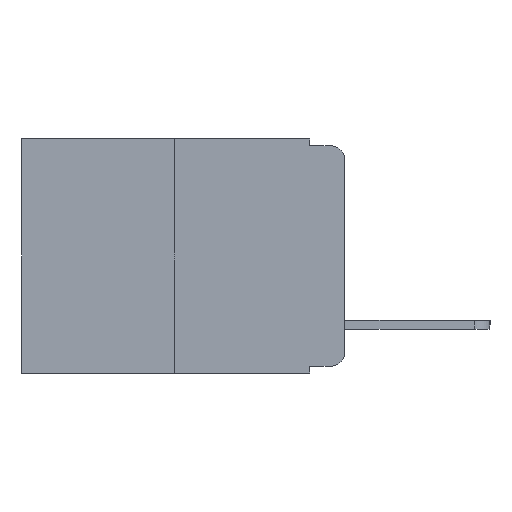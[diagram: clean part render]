
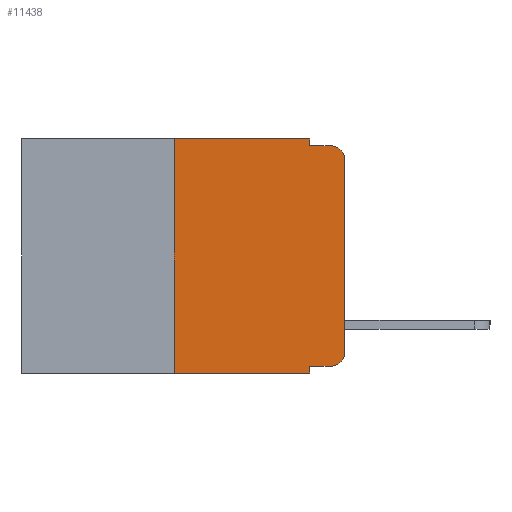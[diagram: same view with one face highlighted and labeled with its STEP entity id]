
A CAD part, left-side view. The second image highlights one B-rep face of the part: STEP entity #11438.
In plain terms, the highlighted planar face has unit normal (-1, 0, 0).
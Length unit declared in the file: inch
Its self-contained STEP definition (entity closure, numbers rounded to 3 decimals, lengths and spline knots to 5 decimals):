
#433 = VECTOR ( 'NONE', #11348, 39.37008 ) ;
#509 = EDGE_CURVE ( 'NONE', #7870, #17186, #17037, .T. ) ;
#562 = DIRECTION ( 'NONE',  ( 1., 0., 0. ) ) ;
#704 = CIRCLE ( 'NONE', #13982, 0.02 ) ;
#1509 = ORIENTED_EDGE ( 'NONE', *, *, #8941, .T. ) ;
#1517 = CARTESIAN_POINT ( 'NONE',  ( 0., 0.02, -0.01 ) ) ;
#1618 = VERTEX_POINT ( 'NONE', #3531 ) ;
#2184 = EDGE_CURVE ( 'NONE', #19096, #15595, #4256, .T. ) ;
#2338 = LINE ( 'NONE', #8220, #433 ) ;
#2557 = CIRCLE ( 'NONE', #18669, 0.02 ) ;
#2660 = ORIENTED_EDGE ( 'NONE', *, *, #10754, .T. ) ;
#2706 = DIRECTION ( 'NONE',  ( 0., 0., -1. ) ) ;
#2711 = DIRECTION ( 'NONE',  ( 0., -1., 0. ) ) ;
#2791 = DIRECTION ( 'NONE',  ( 0., 0., 1. ) ) ;
#3133 = CARTESIAN_POINT ( 'NONE',  ( 0., 0.02, -0.333 ) ) ;
#3222 = ORIENTED_EDGE ( 'NONE', *, *, #9982, .F. ) ;
#3231 = EDGE_LOOP ( 'NONE', ( #7113, #1509, #3222, #7256, #16178, #8993, #17573, #10993, #18399, #2660 ) ) ;
#3531 = CARTESIAN_POINT ( 'NONE',  ( 0., 0.25, 0. ) ) ;
#3757 = DIRECTION ( 'NONE',  ( -1., 0., 0. ) ) ;
#3844 = CARTESIAN_POINT ( 'NONE',  ( 0., 0., -0.313 ) ) ;
#4164 = CARTESIAN_POINT ( 'NONE',  ( 0., 0.051, 0. ) ) ;
#4256 = LINE ( 'NONE', #4164, #17689 ) ;
#5127 = CARTESIAN_POINT ( 'NONE',  ( 0., 0.051, -0.333 ) ) ;
#5367 = VECTOR ( 'NONE', #2711, 39.37008 ) ;
#5397 = DIRECTION ( 'NONE',  ( 0., 0., -1. ) ) ;
#5529 = VERTEX_POINT ( 'NONE', #8472 ) ;
#5745 = DIRECTION ( 'NONE',  ( 0., -1., 0. ) ) ;
#5882 = CARTESIAN_POINT ( 'NONE',  ( 0., 0.473, -0.343 ) ) ;
#6227 = EDGE_CURVE ( 'NONE', #19096, #7724, #18229, .T. ) ;
#6807 = PLANE ( 'NONE',  #12780 ) ;
#7066 = LINE ( 'NONE', #5882, #7161 ) ;
#7113 = ORIENTED_EDGE ( 'NONE', *, *, #8468, .T. ) ;
#7161 = VECTOR ( 'NONE', #17701, 39.37008 ) ;
#7256 = ORIENTED_EDGE ( 'NONE', *, *, #509, .F. ) ;
#7286 = EDGE_CURVE ( 'NONE', #5529, #1618, #14494, .T. ) ;
#7724 = VERTEX_POINT ( 'NONE', #3133 ) ;
#7870 = VERTEX_POINT ( 'NONE', #9610 ) ;
#7988 = CARTESIAN_POINT ( 'NONE',  ( 0., 0.051, -0.343 ) ) ;
#8220 = CARTESIAN_POINT ( 'NONE',  ( 0., 0., 0. ) ) ;
#8468 = EDGE_CURVE ( 'NONE', #18388, #15773, #2338, .T. ) ;
#8472 = CARTESIAN_POINT ( 'NONE',  ( 0., 0.25, -0.343 ) ) ;
#8941 = EDGE_CURVE ( 'NONE', #15773, #18026, #2557, .T. ) ;
#8993 = ORIENTED_EDGE ( 'NONE', *, *, #7286, .F. ) ;
#9353 = CARTESIAN_POINT ( 'NONE',  ( 0., 0.051, -0.333 ) ) ;
#9610 = CARTESIAN_POINT ( 'NONE',  ( 0., 0.051, 0. ) ) ;
#9982 = EDGE_CURVE ( 'NONE', #17186, #18026, #14540, .T. ) ;
#10193 = CARTESIAN_POINT ( 'NONE',  ( 0., 0.051, -0.01 ) ) ;
#10754 = EDGE_CURVE ( 'NONE', #7724, #18388, #704, .T. ) ;
#10816 = EDGE_CURVE ( 'NONE', #5529, #15595, #7066, .T. ) ;
#10993 = ORIENTED_EDGE ( 'NONE', *, *, #2184, .F. ) ;
#11017 = CARTESIAN_POINT ( 'NONE',  ( 0., 0.473, 0. ) ) ;
#11158 = DIRECTION ( 'NONE',  ( 0., 0., -1. ) ) ;
#11348 = DIRECTION ( 'NONE',  ( 0., 0., 1. ) ) ;
#11438 = ADVANCED_FACE ( 'NONE', ( #15729 ), #6807, .F. ) ;
#11627 = CARTESIAN_POINT ( 'NONE',  ( 0., 0.473, 0. ) ) ;
#12260 = DIRECTION ( 'NONE',  ( 0., -1., 0. ) ) ;
#12612 = VECTOR ( 'NONE', #12260, 39.37008 ) ;
#12780 = AXIS2_PLACEMENT_3D ( 'NONE', #11017, #562, #15457 ) ;
#12919 = CARTESIAN_POINT ( 'NONE',  ( 0., 0., -0.03 ) ) ;
#13141 = CARTESIAN_POINT ( 'NONE',  ( 0., 0.051, -0.01 ) ) ;
#13172 = DIRECTION ( 'NONE',  ( 0., 0., -1. ) ) ;
#13982 = AXIS2_PLACEMENT_3D ( 'NONE', #14609, #14409, #13172 ) ;
#14409 = DIRECTION ( 'NONE',  ( -1., 0., 0. ) ) ;
#14494 = LINE ( 'NONE', #17504, #18086 ) ;
#14540 = LINE ( 'NONE', #10193, #17662 ) ;
#14609 = CARTESIAN_POINT ( 'NONE',  ( 0., 0.02, -0.313 ) ) ;
#15457 = DIRECTION ( 'NONE',  ( 0., 0., -1. ) ) ;
#15595 = VERTEX_POINT ( 'NONE', #7988 ) ;
#15729 = FACE_OUTER_BOUND ( 'NONE', #3231, .T. ) ;
#15773 = VERTEX_POINT ( 'NONE', #12919 ) ;
#16055 = LINE ( 'NONE', #11627, #5367 ) ;
#16178 = ORIENTED_EDGE ( 'NONE', *, *, #18757, .F. ) ;
#16862 = CARTESIAN_POINT ( 'NONE',  ( 0., 0.051, 0. ) ) ;
#17037 = LINE ( 'NONE', #16862, #18315 ) ;
#17186 = VERTEX_POINT ( 'NONE', #13141 ) ;
#17504 = CARTESIAN_POINT ( 'NONE',  ( 0., 0.25, 0. ) ) ;
#17573 = ORIENTED_EDGE ( 'NONE', *, *, #10816, .T. ) ;
#17662 = VECTOR ( 'NONE', #5745, 39.37008 ) ;
#17689 = VECTOR ( 'NONE', #2706, 39.37008 ) ;
#17701 = DIRECTION ( 'NONE',  ( 0., -1., 0. ) ) ;
#18026 = VERTEX_POINT ( 'NONE', #1517 ) ;
#18086 = VECTOR ( 'NONE', #2791, 39.37008 ) ;
#18229 = LINE ( 'NONE', #9353, #12612 ) ;
#18315 = VECTOR ( 'NONE', #11158, 39.37008 ) ;
#18388 = VERTEX_POINT ( 'NONE', #3844 ) ;
#18399 = ORIENTED_EDGE ( 'NONE', *, *, #6227, .T. ) ;
#18466 = CARTESIAN_POINT ( 'NONE',  ( 0., 0.02, -0.03 ) ) ;
#18669 = AXIS2_PLACEMENT_3D ( 'NONE', #18466, #3757, #5397 ) ;
#18757 = EDGE_CURVE ( 'NONE', #1618, #7870, #16055, .T. ) ;
#19096 = VERTEX_POINT ( 'NONE', #5127 ) ;
